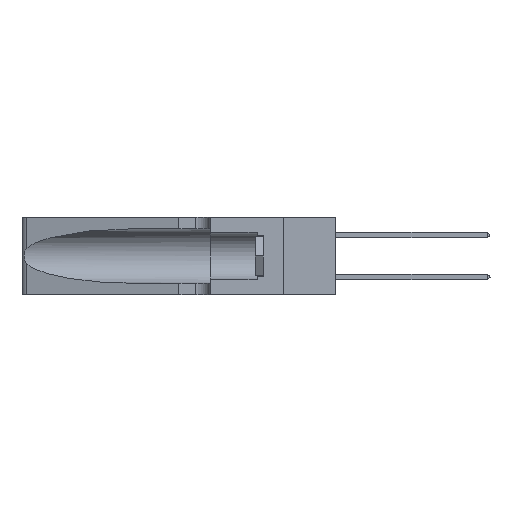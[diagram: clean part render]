
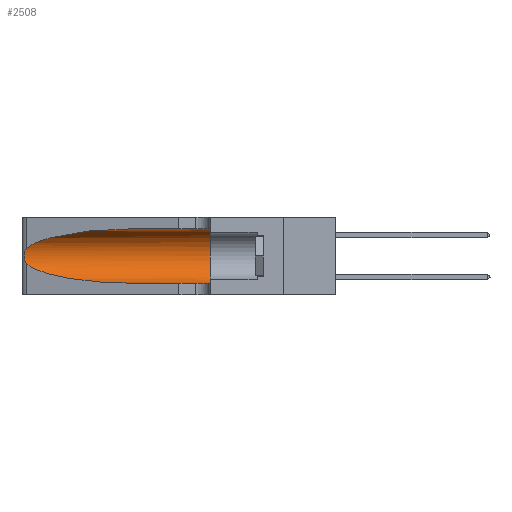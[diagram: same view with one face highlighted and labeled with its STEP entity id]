
A CAD part, left-side view. The second image highlights one B-rep face of the part: STEP entity #2508.
In plain terms, the highlighted cylindrical face has radius 3.308 mm (diameter 6.617 mm), a partial arc.
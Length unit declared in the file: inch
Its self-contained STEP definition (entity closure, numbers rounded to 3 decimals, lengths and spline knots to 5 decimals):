
#2508 = ADVANCED_FACE ( 'NONE', ( #23451 ), #30269, .F. ) ;
#2655 = CARTESIAN_POINT ( 'NONE',  ( 0.25854, 1.2359, 0.20912 ) ) ;
#3422 = ORIENTED_EDGE ( 'NONE', *, *, #3937, .F. ) ;
#3937 = EDGE_CURVE ( 'NONE', #20551, #18922, #25566, .T. ) ;
#4240 = AXIS2_PLACEMENT_3D ( 'NONE', #23926, #34830, #16829 ) ;
#5996 =( BOUNDED_CURVE ( )  B_SPLINE_CURVE ( 3, ( #21752, #7412, #32978, #43546 ),
 .UNSPECIFIED., .F., .F. ) 
 B_SPLINE_CURVE_WITH_KNOTS ( ( 4, 4 ),
 ( 1.5708, 2.84003 ),
 .UNSPECIFIED. ) 
 CURVE ( )  GEOMETRIC_REPRESENTATION_ITEM ( )  RATIONAL_B_SPLINE_CURVE ( ( 1., 0.87, 0.87, 1. ) ) 
 REPRESENTATION_ITEM ( '' )  );
#6001 = CARTESIAN_POINT ( 'NONE',  ( 0.25789, 1.23486, 0.15765 ) ) ;
#7412 = CARTESIAN_POINT ( 'NONE',  ( 0.18966, 0.96281, 0.31525 ) ) ;
#7515 = VECTOR ( 'NONE', #7817, 39.37008 ) ;
#7817 = DIRECTION ( 'NONE',  ( 0., -1., 0. ) ) ;
#9795 = CARTESIAN_POINT ( 'NONE',  ( 0.25555, 1.22994, 0.2215 ) ) ;
#10832 = VERTEX_POINT ( 'NONE', #40059 ) ;
#11049 = VERTEX_POINT ( 'NONE', #19828 ) ;
#12971 = CARTESIAN_POINT ( 'NONE',  ( 0.1305, 1.61858, 0.05475 ) ) ;
#13617 = EDGE_CURVE ( 'NONE', #10832, #24214, #16177, .T. ) ;
#13730 = CARTESIAN_POINT ( 'NONE',  ( 0.25639, 1.23184, 0.21858 ) ) ;
#14424 = EDGE_CURVE ( 'NONE', #18922, #24214, #26235, .T. ) ;
#15374 = CARTESIAN_POINT ( 'NONE',  ( 0.1305, 0.35, 0.31525 ) ) ;
#16177 = LINE ( 'NONE', #12971, #36499 ) ;
#16285 = DIRECTION ( 'NONE',  ( 0., -1., 0. ) ) ;
#16829 = DIRECTION ( 'NONE',  ( 0., 0., -1. ) ) ;
#17079 = CARTESIAN_POINT ( 'NONE',  ( 0.25487, 1.22718, 0.14631 ) ) ;
#17210 = CARTESIAN_POINT ( 'NONE',  ( 0.26075, 1.23896, 0.178 ) ) ;
#18836 = CARTESIAN_POINT ( 'NONE',  ( 0.25487, 1.22718, 0.22369 ) ) ;
#18922 = VERTEX_POINT ( 'NONE', #15374 ) ;
#19828 = CARTESIAN_POINT ( 'NONE',  ( 0.25487, 1.22718, 0.14631 ) ) ;
#20551 = VERTEX_POINT ( 'NONE', #31046 ) ;
#21752 = CARTESIAN_POINT ( 'NONE',  ( 0.1305, 0.72297, 0.31525 ) ) ;
#23451 = FACE_OUTER_BOUND ( 'NONE', #28602, .T. ) ;
#23473 = CARTESIAN_POINT ( 'NONE',  ( 0.1305, 0.35, 0.185 ) ) ;
#23926 = CARTESIAN_POINT ( 'NONE',  ( 0.1305, 1.61858, 0.185 ) ) ;
#24137 = CARTESIAN_POINT ( 'NONE',  ( 0.25487, 1.22718, 0.14631 ) ) ;
#24214 = VERTEX_POINT ( 'NONE', #45153 ) ;
#24291 = CARTESIAN_POINT ( 'NONE',  ( 0.25487, 1.22718, 0.22369 ) ) ;
#24617 = CARTESIAN_POINT ( 'NONE',  ( 0.1305, 0.72297, 0.05475 ) ) ;
#25451 = EDGE_CURVE ( 'NONE', #20551, #37254, #5996, .T. ) ;
#25566 = LINE ( 'NONE', #25807, #7515 ) ;
#25807 = CARTESIAN_POINT ( 'NONE',  ( 0.1305, 1.61858, 0.31525 ) ) ;
#26235 = CIRCLE ( 'NONE', #38082, 0.13025 ) ;
#27112 = DIRECTION ( 'NONE',  ( 0., 1., 0. ) ) ;
#27931 = CARTESIAN_POINT ( 'NONE',  ( 0.26018, 1.23835, 0.19895 ) ) ;
#28236 = CARTESIAN_POINT ( 'NONE',  ( 0.25856, 1.23593, 0.16098 ) ) ;
#28602 = EDGE_LOOP ( 'NONE', ( #41870, #38504, #40796, #34853, #36598, #3422 ) ) ;
#29506 = CARTESIAN_POINT ( 'NONE',  ( 0.18966, 0.96281, 0.05475 ) ) ;
#30269 = CYLINDRICAL_SURFACE ( 'NONE', #4240, 0.13025 ) ;
#30752 = DIRECTION ( 'NONE',  ( 0., 0., 1. ) ) ;
#31046 = CARTESIAN_POINT ( 'NONE',  ( 0.1305, 0.72297, 0.31525 ) ) ;
#31427 = CARTESIAN_POINT ( 'NONE',  ( 0.25639, 1.23186, 0.15144 ) ) ;
#31779 = B_SPLINE_CURVE_WITH_KNOTS ( 'NONE', 3,
 ( #24291, #9795, #13730, #31891, #2655, #27931, #35056, #17210, #38660, #28236, #6001, #31427, #35361, #24137 ),
 .UNSPECIFIED., .F., .F.,
 ( 4, 2, 2, 2, 2, 2, 4 ),
 ( 0., 0.00027, 0.00053, 0.00107, 0.0016, 0.00187, 0.00214 ),
 .UNSPECIFIED. ) ;
#31891 = CARTESIAN_POINT ( 'NONE',  ( 0.25787, 1.23484, 0.2124 ) ) ;
#32978 = CARTESIAN_POINT ( 'NONE',  ( 0.2373, 1.15595, 0.28018 ) ) ;
#34830 = DIRECTION ( 'NONE',  ( 0., -1., 0. ) ) ;
#34853 = ORIENTED_EDGE ( 'NONE', *, *, #13617, .T. ) ;
#35056 = CARTESIAN_POINT ( 'NONE',  ( 0.26075, 1.23896, 0.19203 ) ) ;
#35361 = CARTESIAN_POINT ( 'NONE',  ( 0.25555, 1.22993, 0.14849 ) ) ;
#35739 = EDGE_CURVE ( 'NONE', #11049, #10832, #43626, .T. ) ;
#36499 = VECTOR ( 'NONE', #16285, 39.37008 ) ;
#36598 = ORIENTED_EDGE ( 'NONE', *, *, #14424, .F. ) ;
#37254 = VERTEX_POINT ( 'NONE', #18836 ) ;
#37518 = EDGE_CURVE ( 'NONE', #37254, #11049, #31779, .T. ) ;
#38082 = AXIS2_PLACEMENT_3D ( 'NONE', #23473, #27112, #30752 ) ;
#38504 = ORIENTED_EDGE ( 'NONE', *, *, #37518, .T. ) ;
#38660 = CARTESIAN_POINT ( 'NONE',  ( 0.26017, 1.23833, 0.17102 ) ) ;
#40059 = CARTESIAN_POINT ( 'NONE',  ( 0.1305, 0.72297, 0.05475 ) ) ;
#40796 = ORIENTED_EDGE ( 'NONE', *, *, #35739, .T. ) ;
#41870 = ORIENTED_EDGE ( 'NONE', *, *, #25451, .T. ) ;
#42326 = CARTESIAN_POINT ( 'NONE',  ( 0.2373, 1.15595, 0.08982 ) ) ;
#43546 = CARTESIAN_POINT ( 'NONE',  ( 0.25487, 1.22718, 0.22369 ) ) ;
#43626 =( BOUNDED_CURVE ( )  B_SPLINE_CURVE ( 3, ( #17079, #42326, #29506, #24617 ),
 .UNSPECIFIED., .F., .F. ) 
 B_SPLINE_CURVE_WITH_KNOTS ( ( 4, 4 ),
 ( 3.44316, 4.71239 ),
 .UNSPECIFIED. ) 
 CURVE ( )  GEOMETRIC_REPRESENTATION_ITEM ( )  RATIONAL_B_SPLINE_CURVE ( ( 1., 0.87, 0.87, 1. ) ) 
 REPRESENTATION_ITEM ( '' )  );
#45153 = CARTESIAN_POINT ( 'NONE',  ( 0.1305, 0.35, 0.05475 ) ) ;
